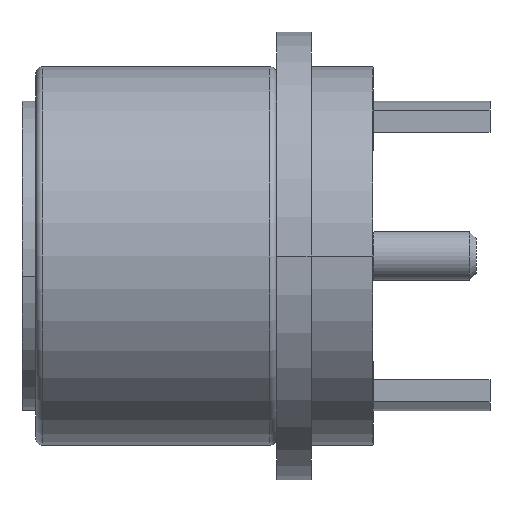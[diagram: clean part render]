
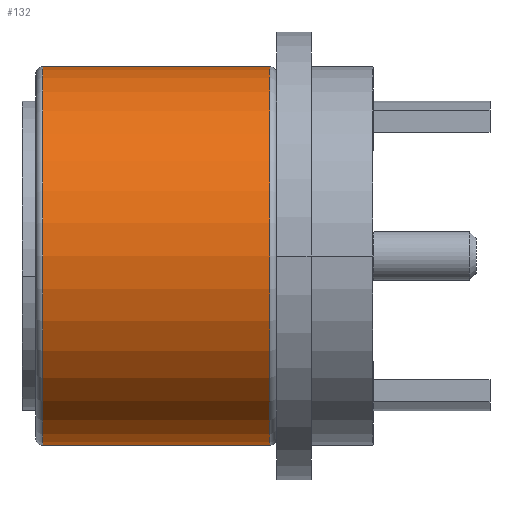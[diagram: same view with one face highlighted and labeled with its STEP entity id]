
A CAD part, left-side view. The second image highlights one B-rep face of the part: STEP entity #132.
In plain terms, the highlighted cylindrical face has radius 2.75 mm (diameter 5.5 mm), a partial arc.
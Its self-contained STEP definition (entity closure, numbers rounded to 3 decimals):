
#28 = AXIS2_PLACEMENT_3D ( 'NONE', #182, #1220, #1045 ) ;
#132 = ADVANCED_FACE ( 'NONE', ( #915 ), #951, .T. ) ;
#182 = CARTESIAN_POINT ( 'NONE',  ( 0., 1.5, 0. ) ) ;
#221 = CARTESIAN_POINT ( 'NONE',  ( 0., 1.5, -2.75 ) ) ;
#254 = DIRECTION ( 'NONE',  ( 0., 0., 1. ) ) ;
#344 = ORIENTED_EDGE ( 'NONE', *, *, #1214, .F. ) ;
#345 = LINE ( 'NONE', #221, #1658 ) ;
#396 = EDGE_CURVE ( 'NONE', #1333, #620, #1422, .T. ) ;
#418 = ORIENTED_EDGE ( 'NONE', *, *, #1626, .T. ) ;
#445 = CARTESIAN_POINT ( 'NONE',  ( 0., 1.434, 0. ) ) ;
#529 = AXIS2_PLACEMENT_3D ( 'NONE', #445, #535, #254 ) ;
#535 = DIRECTION ( 'NONE',  ( 0., 1., 0. ) ) ;
#573 = CARTESIAN_POINT ( 'NONE',  ( 0., 4.8, -2.75 ) ) ;
#575 = VERTEX_POINT ( 'NONE', #573 ) ;
#584 = CIRCLE ( 'NONE', #28, 2.75 ) ;
#620 = VERTEX_POINT ( 'NONE', #1380 ) ;
#730 = VERTEX_POINT ( 'NONE', #1740 ) ;
#915 = FACE_OUTER_BOUND ( 'NONE', #1429, .T. ) ;
#951 = CYLINDRICAL_SURFACE ( 'NONE', #529, 2.75 ) ;
#1045 = DIRECTION ( 'NONE',  ( 0., 0., -1. ) ) ;
#1048 = VECTOR ( 'NONE', #1709, 1000. ) ;
#1214 = EDGE_CURVE ( 'NONE', #730, #575, #345, .T. ) ;
#1220 = DIRECTION ( 'NONE',  ( 0., 1., 0. ) ) ;
#1301 = CIRCLE ( 'NONE', #1406, 2.75 ) ;
#1333 = VERTEX_POINT ( 'NONE', #1545 ) ;
#1334 = ORIENTED_EDGE ( 'NONE', *, *, #396, .F. ) ;
#1380 = CARTESIAN_POINT ( 'NONE',  ( 0., 1.5, 2.75 ) ) ;
#1406 = AXIS2_PLACEMENT_3D ( 'NONE', #1656, #1460, #1811 ) ;
#1422 = LINE ( 'NONE', #1742, #1048 ) ;
#1425 = ORIENTED_EDGE ( 'NONE', *, *, #1733, .T. ) ;
#1429 = EDGE_LOOP ( 'NONE', ( #418, #1334, #1425, #344 ) ) ;
#1460 = DIRECTION ( 'NONE',  ( 0., -1., 0. ) ) ;
#1545 = CARTESIAN_POINT ( 'NONE',  ( 0., 4.8, 2.75 ) ) ;
#1626 = EDGE_CURVE ( 'NONE', #730, #620, #584, .T. ) ;
#1656 = CARTESIAN_POINT ( 'NONE',  ( 0., 4.8, 0. ) ) ;
#1658 = VECTOR ( 'NONE', #1757, 1000. ) ;
#1709 = DIRECTION ( 'NONE',  ( 0., -1., 0. ) ) ;
#1733 = EDGE_CURVE ( 'NONE', #1333, #575, #1301, .T. ) ;
#1740 = CARTESIAN_POINT ( 'NONE',  ( 0., 1.5, -2.75 ) ) ;
#1742 = CARTESIAN_POINT ( 'NONE',  ( 0., 4.8, 2.75 ) ) ;
#1757 = DIRECTION ( 'NONE',  ( 0., 1., 0. ) ) ;
#1811 = DIRECTION ( 'NONE',  ( 0., 0., 1. ) ) ;
